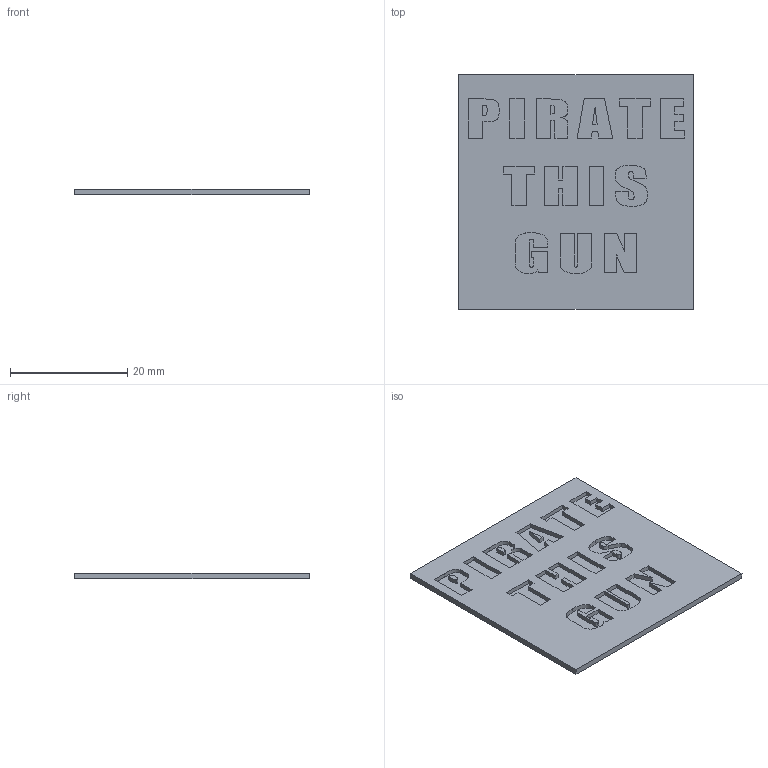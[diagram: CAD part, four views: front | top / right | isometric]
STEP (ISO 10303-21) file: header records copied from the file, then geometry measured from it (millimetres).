
FILE_DESCRIPTION (( 'STEP AP214' ), '1' );
FILE_NAME ('Pirate_This_Gun.STEP', '2013-09-01T16:53:19', ( 'Asher' ), ( '' ), 'SwSTEP 2.0', 'SolidWorks 2013', '' );
FILE_SCHEMA (( 'AUTOMOTIVE_DESIGN' ));
Length unit declared in the file: millimetre
Products named in the file (1): Pirate_This_Gun
Bounding box: 40 x 40 x 1 mm (x, y, z)
Volume: 1345.8 mm3; surface area: 3647.3 mm2
Topology: 1 solids, 1 shells, 170 faces, 456 edges, 304 vertices
Faces by surface type: plane 130, bspline 40
Entity records: 7769 total; most frequent: CARTESIAN_POINT 3603, ORIENTED_EDGE 912, DIRECTION 638, EDGE_CURVE 456, LINE 376, VECTOR 376, VERTEX_POINT 304, EDGE_LOOP 186
